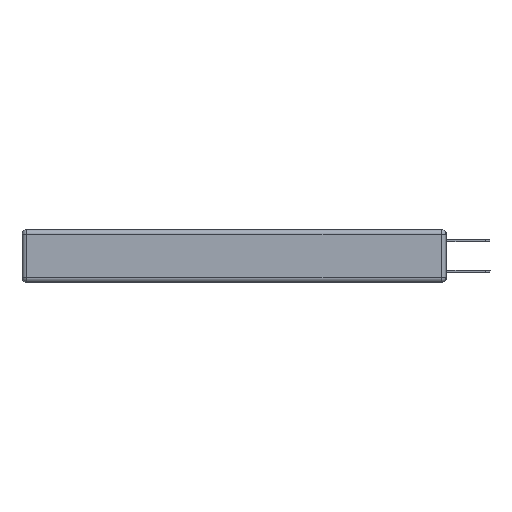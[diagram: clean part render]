
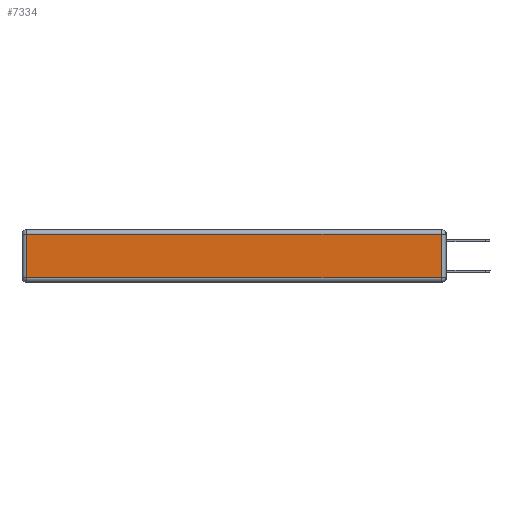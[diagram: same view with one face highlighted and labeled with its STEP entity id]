
A CAD part, left-side view. The second image highlights one B-rep face of the part: STEP entity #7334.
In plain terms, the highlighted planar face has unit normal (-1, 0, 0).
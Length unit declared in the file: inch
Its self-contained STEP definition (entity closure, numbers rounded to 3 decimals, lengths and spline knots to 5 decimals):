
#302 = DIRECTION ( 'NONE',  ( 0., 0., -1. ) ) ;
#308 = CARTESIAN_POINT ( 'NONE',  ( 0., 2.72, -0.03 ) ) ;
#500 = EDGE_LOOP ( 'NONE', ( #2915, #11405, #7774, #1342 ) ) ;
#1188 = LINE ( 'NONE', #6898, #6967 ) ;
#1230 = FACE_OUTER_BOUND ( 'NONE', #500, .T. ) ;
#1342 = ORIENTED_EDGE ( 'NONE', *, *, #2500, .T. ) ;
#2003 = VECTOR ( 'NONE', #11215, 39.37008 ) ;
#2500 = EDGE_CURVE ( 'NONE', #10812, #3591, #1188, .T. ) ;
#2915 = ORIENTED_EDGE ( 'NONE', *, *, #8365, .T. ) ;
#3150 = CARTESIAN_POINT ( 'NONE',  ( 0., 0.03, -0.343 ) ) ;
#3275 = LINE ( 'NONE', #3150, #8473 ) ;
#3591 = VERTEX_POINT ( 'NONE', #8494 ) ;
#4234 = DIRECTION ( 'NONE',  ( 0., -1., 0. ) ) ;
#5176 = LINE ( 'NONE', #9068, #7470 ) ;
#5271 = PLANE ( 'NONE',  #7302 ) ;
#5972 = DIRECTION ( 'NONE',  ( -1., 0., 0. ) ) ;
#6265 = VERTEX_POINT ( 'NONE', #6602 ) ;
#6512 = VERTEX_POINT ( 'NONE', #10916 ) ;
#6602 = CARTESIAN_POINT ( 'NONE',  ( 0., 0.03, -0.313 ) ) ;
#6898 = CARTESIAN_POINT ( 'NONE',  ( 0., 2.72, -0.343 ) ) ;
#6967 = VECTOR ( 'NONE', #302, 39.37008 ) ;
#7032 = DIRECTION ( 'NONE',  ( 0., 0., 1. ) ) ;
#7302 = AXIS2_PLACEMENT_3D ( 'NONE', #9101, #5972, #8070 ) ;
#7334 = ADVANCED_FACE ( 'NONE', ( #1230 ), #5271, .T. ) ;
#7470 = VECTOR ( 'NONE', #4234, 39.37008 ) ;
#7774 = ORIENTED_EDGE ( 'NONE', *, *, #8420, .T. ) ;
#8070 = DIRECTION ( 'NONE',  ( 0., 0., 1. ) ) ;
#8365 = EDGE_CURVE ( 'NONE', #3591, #6265, #5176, .T. ) ;
#8420 = EDGE_CURVE ( 'NONE', #6512, #10812, #11334, .T. ) ;
#8473 = VECTOR ( 'NONE', #7032, 39.37008 ) ;
#8494 = CARTESIAN_POINT ( 'NONE',  ( 0., 2.72, -0.313 ) ) ;
#9068 = CARTESIAN_POINT ( 'NONE',  ( 0., 0., -0.313 ) ) ;
#9101 = CARTESIAN_POINT ( 'NONE',  ( 0., 0., -0.343 ) ) ;
#9134 = CARTESIAN_POINT ( 'NONE',  ( 0., 2.75, -0.03 ) ) ;
#9658 = EDGE_CURVE ( 'NONE', #6265, #6512, #3275, .T. ) ;
#10812 = VERTEX_POINT ( 'NONE', #308 ) ;
#10916 = CARTESIAN_POINT ( 'NONE',  ( 0., 0.03, -0.03 ) ) ;
#11215 = DIRECTION ( 'NONE',  ( 0., 1., 0. ) ) ;
#11334 = LINE ( 'NONE', #9134, #2003 ) ;
#11405 = ORIENTED_EDGE ( 'NONE', *, *, #9658, .T. ) ;
